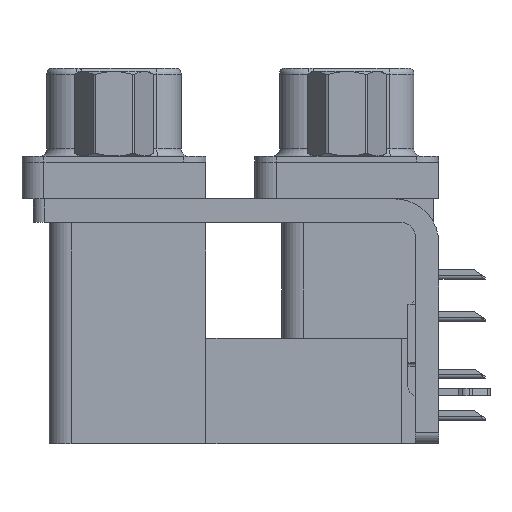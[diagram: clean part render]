
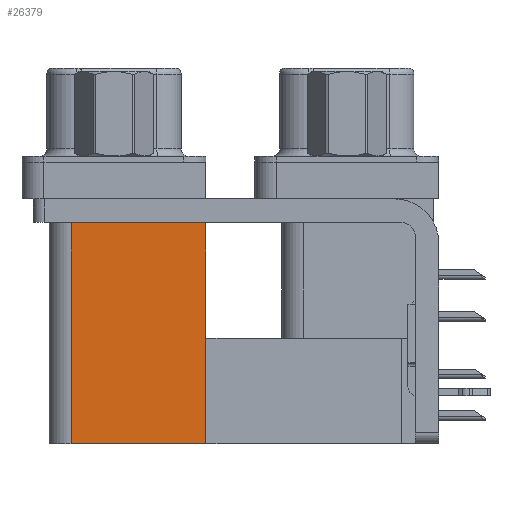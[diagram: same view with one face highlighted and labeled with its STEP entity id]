
A CAD part, left-side view. The second image highlights one B-rep face of the part: STEP entity #26379.
In plain terms, the highlighted planar face has unit normal (-1, 0, 0).
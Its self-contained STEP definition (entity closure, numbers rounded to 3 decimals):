
#3419 = PLANE ( 'NONE',  #23880 ) ;
#3725 = DIRECTION ( 'NONE',  ( 0., 0., 1. ) ) ;
#3806 = ORIENTED_EDGE ( 'NONE', *, *, #14487, .T. ) ;
#4458 = LINE ( 'NONE', #28158, #34054 ) ;
#5788 = CARTESIAN_POINT ( 'NONE',  ( 3.765, 9.6, -19.2 ) ) ;
#6034 = VECTOR ( 'NONE', #3725, 1000. ) ;
#6711 = CARTESIAN_POINT ( 'NONE',  ( 3.765, 9.6, -19.2 ) ) ;
#7515 = CARTESIAN_POINT ( 'NONE',  ( 3.765, 9.6, -2.5 ) ) ;
#7518 = VERTEX_POINT ( 'NONE', #30154 ) ;
#7821 = EDGE_CURVE ( 'NONE', #34051, #7518, #4458, .T. ) ;
#8718 = LINE ( 'NONE', #21043, #21197 ) ;
#9151 = VECTOR ( 'NONE', #14380, 1000. ) ;
#12865 = DIRECTION ( 'NONE',  ( 1., 0., 0. ) ) ;
#14380 = DIRECTION ( 'NONE',  ( 0., 1., 0. ) ) ;
#14487 = EDGE_CURVE ( 'NONE', #27644, #34051, #30115, .T. ) ;
#19473 = VERTEX_POINT ( 'NONE', #37385 ) ;
#21043 = CARTESIAN_POINT ( 'NONE',  ( 3.765, 18.8, -19.2 ) ) ;
#21197 = VECTOR ( 'NONE', #29492, 1000. ) ;
#23843 = DIRECTION ( 'NONE',  ( 0., 0., -1. ) ) ;
#23880 = AXIS2_PLACEMENT_3D ( 'NONE', #6711, #12865, #23843 ) ;
#26158 = FACE_OUTER_BOUND ( 'NONE', #34783, .T. ) ;
#26379 = ADVANCED_FACE ( 'NONE', ( #26158 ), #3419, .F. ) ;
#26570 = EDGE_CURVE ( 'NONE', #27644, #19473, #28620, .T. ) ;
#27644 = VERTEX_POINT ( 'NONE', #5788 ) ;
#28158 = CARTESIAN_POINT ( 'NONE',  ( 3.765, 9.6, -2.5 ) ) ;
#28479 = ORIENTED_EDGE ( 'NONE', *, *, #26570, .F. ) ;
#28525 = DIRECTION ( 'NONE',  ( 0., 1., 0. ) ) ;
#28620 = LINE ( 'NONE', #37836, #9151 ) ;
#28652 = ORIENTED_EDGE ( 'NONE', *, *, #37664, .F. ) ;
#29492 = DIRECTION ( 'NONE',  ( 0., 0., 1. ) ) ;
#30115 = LINE ( 'NONE', #35106, #6034 ) ;
#30154 = CARTESIAN_POINT ( 'NONE',  ( 3.765, 18.8, -2.5 ) ) ;
#34051 = VERTEX_POINT ( 'NONE', #7515 ) ;
#34054 = VECTOR ( 'NONE', #28525, 1000. ) ;
#34783 = EDGE_LOOP ( 'NONE', ( #38058, #28652, #28479, #3806 ) ) ;
#35106 = CARTESIAN_POINT ( 'NONE',  ( 3.765, 9.6, -19.2 ) ) ;
#37385 = CARTESIAN_POINT ( 'NONE',  ( 3.765, 18.8, -19.2 ) ) ;
#37664 = EDGE_CURVE ( 'NONE', #19473, #7518, #8718, .T. ) ;
#37836 = CARTESIAN_POINT ( 'NONE',  ( 3.765, 9.6, -19.2 ) ) ;
#38058 = ORIENTED_EDGE ( 'NONE', *, *, #7821, .T. ) ;
